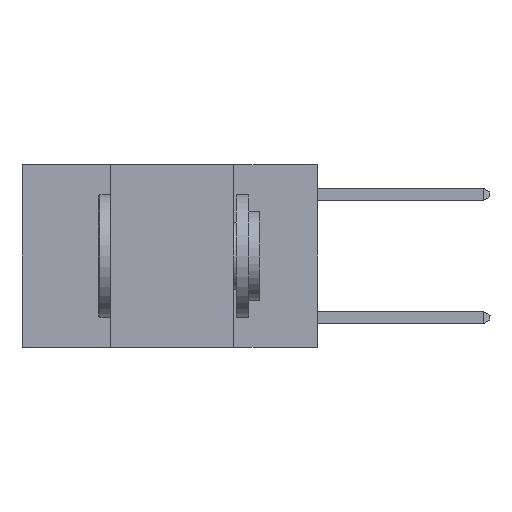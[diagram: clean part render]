
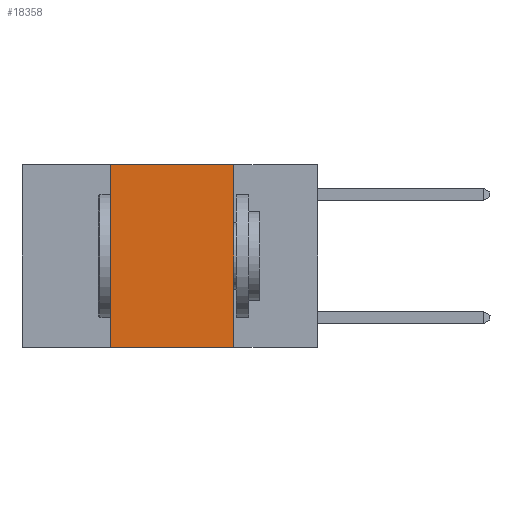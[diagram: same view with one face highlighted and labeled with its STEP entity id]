
A CAD part, left-side view. The second image highlights one B-rep face of the part: STEP entity #18358.
In plain terms, the highlighted planar face has unit normal (-1, 0, 0).
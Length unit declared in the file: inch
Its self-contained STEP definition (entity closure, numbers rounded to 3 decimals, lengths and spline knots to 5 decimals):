
#379 = CARTESIAN_POINT ( 'NONE',  ( 0., 0.17, 0. ) ) ;
#716 = VERTEX_POINT ( 'NONE', #14328 ) ;
#755 = VECTOR ( 'NONE', #15617, 39.37008 ) ;
#1546 = EDGE_CURVE ( 'NONE', #4764, #716, #3665, .T. ) ;
#2333 = EDGE_LOOP ( 'NONE', ( #6236, #8014, #17855, #20084 ) ) ;
#2523 = DIRECTION ( 'NONE',  ( 0., 0., 1. ) ) ;
#2661 = CARTESIAN_POINT ( 'NONE',  ( 0., 0.42, 0. ) ) ;
#3344 = VECTOR ( 'NONE', #14716, 39.37008 ) ;
#3600 = VERTEX_POINT ( 'NONE', #8298 ) ;
#3665 = LINE ( 'NONE', #2661, #11672 ) ;
#3666 = EDGE_CURVE ( 'NONE', #12177, #3600, #16483, .T. ) ;
#4764 = VERTEX_POINT ( 'NONE', #18831 ) ;
#6236 = ORIENTED_EDGE ( 'NONE', *, *, #3666, .F. ) ;
#7026 = CARTESIAN_POINT ( 'NONE',  ( 0., 0.6, -0.37 ) ) ;
#8014 = ORIENTED_EDGE ( 'NONE', *, *, #18675, .F. ) ;
#8298 = CARTESIAN_POINT ( 'NONE',  ( 0., 0.17, -0.37 ) ) ;
#8519 = DIRECTION ( 'NONE',  ( 1., 0., 0. ) ) ;
#8637 = DIRECTION ( 'NONE',  ( 0., -1., 0. ) ) ;
#8655 = AXIS2_PLACEMENT_3D ( 'NONE', #11656, #8519, #19487 ) ;
#9882 = CARTESIAN_POINT ( 'NONE',  ( 0., 0.17, 0. ) ) ;
#11421 = VECTOR ( 'NONE', #8637, 39.37008 ) ;
#11656 = CARTESIAN_POINT ( 'NONE',  ( 0., 0.6, 0. ) ) ;
#11672 = VECTOR ( 'NONE', #2523, 39.37008 ) ;
#12177 = VERTEX_POINT ( 'NONE', #9882 ) ;
#12994 = LINE ( 'NONE', #14053, #755 ) ;
#13667 = EDGE_CURVE ( 'NONE', #4764, #3600, #15102, .T. ) ;
#14053 = CARTESIAN_POINT ( 'NONE',  ( 0., 0.6, 0. ) ) ;
#14328 = CARTESIAN_POINT ( 'NONE',  ( 0., 0.42, 0. ) ) ;
#14716 = DIRECTION ( 'NONE',  ( 0., 0., -1. ) ) ;
#15102 = LINE ( 'NONE', #7026, #11421 ) ;
#15617 = DIRECTION ( 'NONE',  ( 0., -1., 0. ) ) ;
#16483 = LINE ( 'NONE', #379, #3344 ) ;
#17855 = ORIENTED_EDGE ( 'NONE', *, *, #1546, .F. ) ;
#17945 = PLANE ( 'NONE',  #8655 ) ;
#18091 = FACE_OUTER_BOUND ( 'NONE', #2333, .T. ) ;
#18358 = ADVANCED_FACE ( 'NONE', ( #18091 ), #17945, .F. ) ;
#18675 = EDGE_CURVE ( 'NONE', #716, #12177, #12994, .T. ) ;
#18831 = CARTESIAN_POINT ( 'NONE',  ( 0., 0.42, -0.37 ) ) ;
#19487 = DIRECTION ( 'NONE',  ( 0., 0., -1. ) ) ;
#20084 = ORIENTED_EDGE ( 'NONE', *, *, #13667, .T. ) ;
